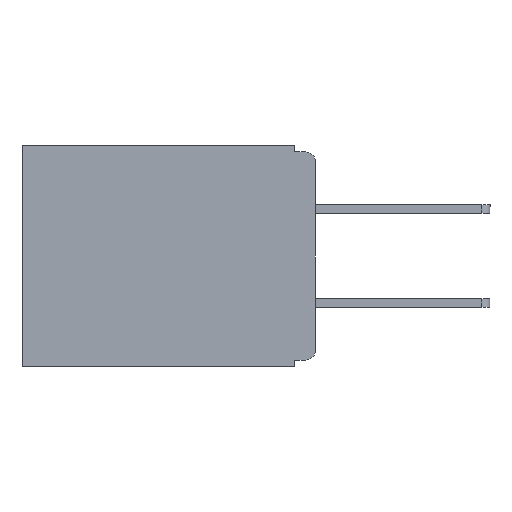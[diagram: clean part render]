
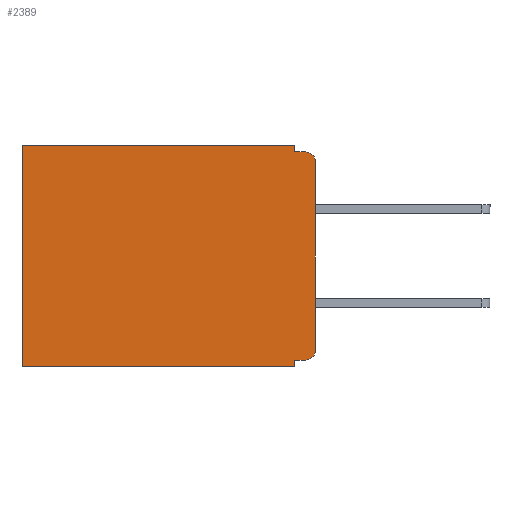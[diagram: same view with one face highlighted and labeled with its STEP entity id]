
A CAD part, left-side view. The second image highlights one B-rep face of the part: STEP entity #2389.
In plain terms, the highlighted planar face has unit normal (-1, 0, 0).
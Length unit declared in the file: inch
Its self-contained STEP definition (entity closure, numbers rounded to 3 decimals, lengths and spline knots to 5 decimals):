
#153 = DIRECTION ( 'NONE',  ( 0., 0., -1. ) ) ;
#588 = ORIENTED_EDGE ( 'NONE', *, *, #5162, .T. ) ;
#733 = LINE ( 'NONE', #1209, #5708 ) ;
#970 = EDGE_CURVE ( 'NONE', #10014, #12338, #7872, .T. ) ;
#1075 = DIRECTION ( 'NONE',  ( 0., 1., 0. ) ) ;
#1174 = CARTESIAN_POINT ( 'NONE',  ( 0.3, 0.015, -0.025 ) ) ;
#1209 = CARTESIAN_POINT ( 'NONE',  ( 0.3, 0., -0.33 ) ) ;
#1238 = CARTESIAN_POINT ( 'NONE',  ( 0.3, 0., -0.33 ) ) ;
#1318 = EDGE_CURVE ( 'NONE', #11248, #10255, #4188, .T. ) ;
#1425 = ORIENTED_EDGE ( 'NONE', *, *, #7775, .F. ) ;
#1497 = LINE ( 'NONE', #4632, #4767 ) ;
#1498 = EDGE_CURVE ( 'NONE', #1553, #9426, #10225, .T. ) ;
#1553 = VERTEX_POINT ( 'NONE', #8003 ) ;
#1759 = AXIS2_PLACEMENT_3D ( 'NONE', #1174, #7101, #153 ) ;
#1863 = CARTESIAN_POINT ( 'NONE',  ( 0.3, 0.437, 0. ) ) ;
#1887 = DIRECTION ( 'NONE',  ( 0., 0., -1. ) ) ;
#1923 = CARTESIAN_POINT ( 'NONE',  ( 0.3, 0.015, -0.32 ) ) ;
#2069 = CARTESIAN_POINT ( 'NONE',  ( 0.3, 0.031, 0. ) ) ;
#2216 = EDGE_CURVE ( 'NONE', #3390, #9426, #10054, .T. ) ;
#2359 = AXIS2_PLACEMENT_3D ( 'NONE', #4886, #8602, #12494 ) ;
#2389 = ADVANCED_FACE ( 'NONE', ( #5524 ), #12715, .F. ) ;
#2564 = VERTEX_POINT ( 'NONE', #2069 ) ;
#2568 = VERTEX_POINT ( 'NONE', #4550 ) ;
#2678 = EDGE_CURVE ( 'NONE', #2564, #3390, #1497, .T. ) ;
#3110 = ORIENTED_EDGE ( 'NONE', *, *, #970, .F. ) ;
#3150 = LINE ( 'NONE', #9755, #11060 ) ;
#3268 = EDGE_LOOP ( 'NONE', ( #1425, #5221, #3325, #10415, #9472, #8853, #11697, #4369, #3110, #588 ) ) ;
#3325 = ORIENTED_EDGE ( 'NONE', *, *, #2216, .F. ) ;
#3390 = VERTEX_POINT ( 'NONE', #6368 ) ;
#3893 = DIRECTION ( 'NONE',  ( -1., 0., 0. ) ) ;
#3901 = DIRECTION ( 'NONE',  ( 0., 0., -1. ) ) ;
#4066 = CARTESIAN_POINT ( 'NONE',  ( 0.3, 0.015, -0.305 ) ) ;
#4113 = AXIS2_PLACEMENT_3D ( 'NONE', #4066, #3893, #3901 ) ;
#4188 = LINE ( 'NONE', #12492, #6774 ) ;
#4369 = ORIENTED_EDGE ( 'NONE', *, *, #7441, .F. ) ;
#4550 = CARTESIAN_POINT ( 'NONE',  ( 0.3, 0., -0.305 ) ) ;
#4632 = CARTESIAN_POINT ( 'NONE',  ( 0.3, 0.031, 0. ) ) ;
#4724 = CARTESIAN_POINT ( 'NONE',  ( 0.3, 0.031, -0.33 ) ) ;
#4767 = VECTOR ( 'NONE', #11577, 39.37008 ) ;
#4886 = CARTESIAN_POINT ( 'NONE',  ( 0.3, 0., -0.33 ) ) ;
#5162 = EDGE_CURVE ( 'NONE', #10014, #2568, #8224, .T. ) ;
#5193 = CARTESIAN_POINT ( 'NONE',  ( 0.3, 0.437, -0.33 ) ) ;
#5221 = ORIENTED_EDGE ( 'NONE', *, *, #1498, .T. ) ;
#5382 = EDGE_CURVE ( 'NONE', #2564, #11248, #3150, .T. ) ;
#5524 = FACE_OUTER_BOUND ( 'NONE', #3268, .T. ) ;
#5708 = VECTOR ( 'NONE', #7137, 39.37008 ) ;
#6368 = CARTESIAN_POINT ( 'NONE',  ( 0.3, 0.031, -0.01 ) ) ;
#6774 = VECTOR ( 'NONE', #7744, 39.37008 ) ;
#6837 = VERTEX_POINT ( 'NONE', #4724 ) ;
#6965 = CARTESIAN_POINT ( 'NONE',  ( 0.3, 0., -0.01 ) ) ;
#6981 = DIRECTION ( 'NONE',  ( 0., -1., 0. ) ) ;
#7101 = DIRECTION ( 'NONE',  ( -1., 0., 0. ) ) ;
#7137 = DIRECTION ( 'NONE',  ( 0., 0., -1. ) ) ;
#7441 = EDGE_CURVE ( 'NONE', #12338, #6837, #12396, .T. ) ;
#7744 = DIRECTION ( 'NONE',  ( 0., 0., -1. ) ) ;
#7775 = EDGE_CURVE ( 'NONE', #1553, #2568, #733, .T. ) ;
#7829 = CARTESIAN_POINT ( 'NONE',  ( 0.3, 0.015, -0.01 ) ) ;
#7872 = LINE ( 'NONE', #9944, #12845 ) ;
#8003 = CARTESIAN_POINT ( 'NONE',  ( 0.3, 0., -0.025 ) ) ;
#8224 = CIRCLE ( 'NONE', #4113, 0.015 ) ;
#8602 = DIRECTION ( 'NONE',  ( 1., 0., 0. ) ) ;
#8736 = DIRECTION ( 'NONE',  ( 0., 1., 0. ) ) ;
#8853 = ORIENTED_EDGE ( 'NONE', *, *, #1318, .T. ) ;
#9424 = CARTESIAN_POINT ( 'NONE',  ( 0.3, 0.031, -0.33 ) ) ;
#9426 = VERTEX_POINT ( 'NONE', #7829 ) ;
#9472 = ORIENTED_EDGE ( 'NONE', *, *, #5382, .T. ) ;
#9755 = CARTESIAN_POINT ( 'NONE',  ( 0.3, 0., 0. ) ) ;
#9777 = VECTOR ( 'NONE', #1887, 39.37008 ) ;
#9944 = CARTESIAN_POINT ( 'NONE',  ( 0.3, 0., -0.32 ) ) ;
#10014 = VERTEX_POINT ( 'NONE', #1923 ) ;
#10054 = LINE ( 'NONE', #6965, #12663 ) ;
#10225 = CIRCLE ( 'NONE', #1759, 0.015 ) ;
#10255 = VERTEX_POINT ( 'NONE', #5193 ) ;
#10415 = ORIENTED_EDGE ( 'NONE', *, *, #2678, .F. ) ;
#10845 = EDGE_CURVE ( 'NONE', #6837, #10255, #11852, .T. ) ;
#11060 = VECTOR ( 'NONE', #8736, 39.37008 ) ;
#11166 = DIRECTION ( 'NONE',  ( 0., 1., 0. ) ) ;
#11248 = VERTEX_POINT ( 'NONE', #1863 ) ;
#11546 = VECTOR ( 'NONE', #11166, 39.37008 ) ;
#11577 = DIRECTION ( 'NONE',  ( 0., 0., -1. ) ) ;
#11679 = CARTESIAN_POINT ( 'NONE',  ( 0.3, 0.031, -0.32 ) ) ;
#11697 = ORIENTED_EDGE ( 'NONE', *, *, #10845, .F. ) ;
#11852 = LINE ( 'NONE', #1238, #11546 ) ;
#12338 = VERTEX_POINT ( 'NONE', #11679 ) ;
#12396 = LINE ( 'NONE', #9424, #9777 ) ;
#12492 = CARTESIAN_POINT ( 'NONE',  ( 0.3, 0.437, -0.33 ) ) ;
#12494 = DIRECTION ( 'NONE',  ( 0., 0., -1. ) ) ;
#12663 = VECTOR ( 'NONE', #6981, 39.37008 ) ;
#12715 = PLANE ( 'NONE',  #2359 ) ;
#12845 = VECTOR ( 'NONE', #1075, 39.37008 ) ;
